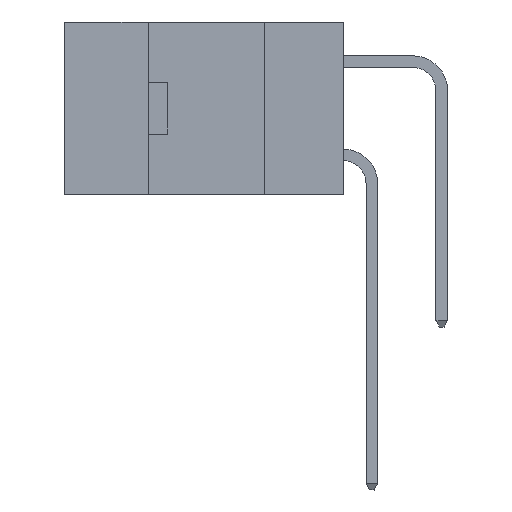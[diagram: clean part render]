
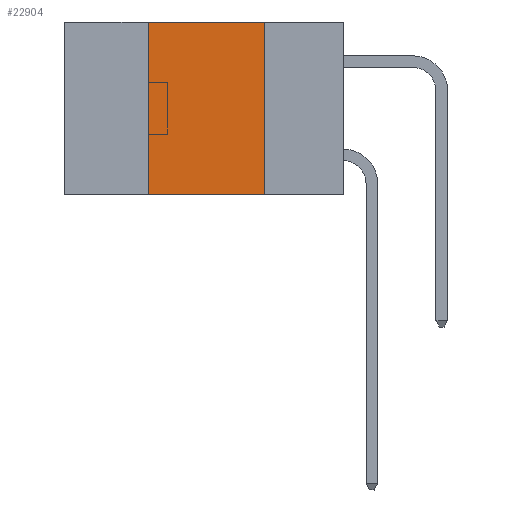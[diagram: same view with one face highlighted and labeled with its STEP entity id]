
A CAD part, left-side view. The second image highlights one B-rep face of the part: STEP entity #22904.
In plain terms, the highlighted planar face has unit normal (-1, 0, 0).
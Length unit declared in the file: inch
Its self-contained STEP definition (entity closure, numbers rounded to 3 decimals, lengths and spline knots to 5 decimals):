
#340 = LINE ( 'NONE', #21775, #1902 ) ;
#502 = VERTEX_POINT ( 'NONE', #20025 ) ;
#672 = VERTEX_POINT ( 'NONE', #27829 ) ;
#981 = CARTESIAN_POINT ( 'NONE',  ( 0., 0.6, 0. ) ) ;
#1018 = PLANE ( 'NONE',  #5087 ) ;
#1193 = DIRECTION ( 'NONE',  ( 0., 0., -1. ) ) ;
#1902 = VECTOR ( 'NONE', #1193, 39.37008 ) ;
#2444 = VERTEX_POINT ( 'NONE', #20748 ) ;
#3048 = ORIENTED_EDGE ( 'NONE', *, *, #10614, .F. ) ;
#3276 = LINE ( 'NONE', #12421, #20647 ) ;
#5087 = AXIS2_PLACEMENT_3D ( 'NONE', #10163, #10308, #22033 ) ;
#5496 = ORIENTED_EDGE ( 'NONE', *, *, #6956, .T. ) ;
#5869 = CARTESIAN_POINT ( 'NONE',  ( 0., 0.6, -0.37 ) ) ;
#6956 = EDGE_CURVE ( 'NONE', #2444, #502, #24498, .T. ) ;
#9477 = VECTOR ( 'NONE', #21937, 39.37008 ) ;
#10124 = DIRECTION ( 'NONE',  ( 0., -1., 0. ) ) ;
#10163 = CARTESIAN_POINT ( 'NONE',  ( 0., 0.6, 0. ) ) ;
#10168 = DIRECTION ( 'NONE',  ( 0., 0., 1. ) ) ;
#10302 = EDGE_CURVE ( 'NONE', #28482, #672, #21560, .T. ) ;
#10308 = DIRECTION ( 'NONE',  ( 1., 0., 0. ) ) ;
#10614 = EDGE_CURVE ( 'NONE', #672, #502, #340, .T. ) ;
#11077 = EDGE_CURVE ( 'NONE', #2444, #28482, #3276, .T. ) ;
#12421 = CARTESIAN_POINT ( 'NONE',  ( 0., 0.42, -0.37 ) ) ;
#17362 = FACE_OUTER_BOUND ( 'NONE', #29499, .T. ) ;
#20025 = CARTESIAN_POINT ( 'NONE',  ( 0., 0.17, -0.37 ) ) ;
#20647 = VECTOR ( 'NONE', #10168, 39.37008 ) ;
#20748 = CARTESIAN_POINT ( 'NONE',  ( 0., 0.42, -0.37 ) ) ;
#21560 = LINE ( 'NONE', #981, #24445 ) ;
#21775 = CARTESIAN_POINT ( 'NONE',  ( 0., 0.17, -0.37 ) ) ;
#21937 = DIRECTION ( 'NONE',  ( 0., -1., 0. ) ) ;
#22033 = DIRECTION ( 'NONE',  ( 0., 0., -1. ) ) ;
#22283 = ORIENTED_EDGE ( 'NONE', *, *, #11077, .F. ) ;
#22904 = ADVANCED_FACE ( 'NONE', ( #17362 ), #1018, .F. ) ;
#24445 = VECTOR ( 'NONE', #10124, 39.37008 ) ;
#24498 = LINE ( 'NONE', #5869, #9477 ) ;
#25137 = ORIENTED_EDGE ( 'NONE', *, *, #10302, .F. ) ;
#27829 = CARTESIAN_POINT ( 'NONE',  ( 0., 0.17, 0. ) ) ;
#28482 = VERTEX_POINT ( 'NONE', #28953 ) ;
#28953 = CARTESIAN_POINT ( 'NONE',  ( 0., 0.42, 0. ) ) ;
#29499 = EDGE_LOOP ( 'NONE', ( #3048, #25137, #22283, #5496 ) ) ;
